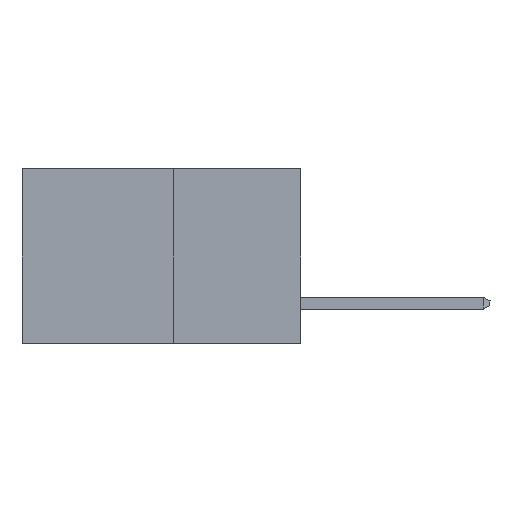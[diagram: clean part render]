
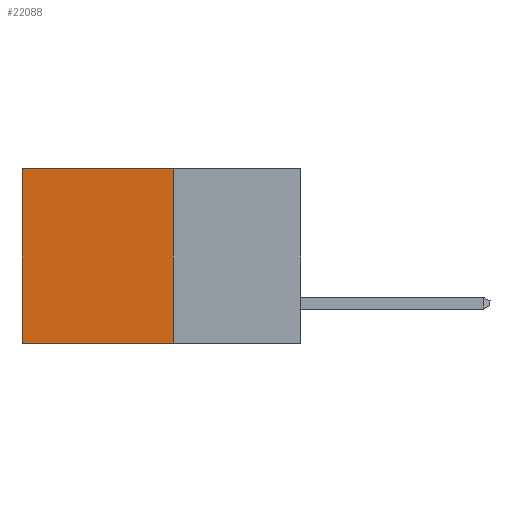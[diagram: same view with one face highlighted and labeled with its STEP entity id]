
A CAD part, left-side view. The second image highlights one B-rep face of the part: STEP entity #22088.
In plain terms, the highlighted planar face has unit normal (-1, 0, 0).
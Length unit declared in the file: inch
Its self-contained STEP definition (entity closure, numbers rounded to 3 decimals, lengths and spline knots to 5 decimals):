
#2346 = DIRECTION ( 'NONE',  ( 0., 0., -1. ) ) ;
#3459 = CARTESIAN_POINT ( 'NONE',  ( 0.277, 0.27, 0. ) ) ;
#5425 = CARTESIAN_POINT ( 'NONE',  ( 0.277, 0.59, -0.37 ) ) ;
#5531 = EDGE_CURVE ( 'NONE', #6152, #24925, #17665, .T. ) ;
#5925 = DIRECTION ( 'NONE',  ( 0., 1., 0. ) ) ;
#6152 = VERTEX_POINT ( 'NONE', #19104 ) ;
#6486 = DIRECTION ( 'NONE',  ( 0., 1., 0. ) ) ;
#6534 = CARTESIAN_POINT ( 'NONE',  ( 0.277, 0.27, -0.37 ) ) ;
#6620 = VERTEX_POINT ( 'NONE', #6926 ) ;
#6926 = CARTESIAN_POINT ( 'NONE',  ( 0.277, 0.59, 0. ) ) ;
#7099 = CARTESIAN_POINT ( 'NONE',  ( 0.277, 0.59, -0.37 ) ) ;
#8309 = CARTESIAN_POINT ( 'NONE',  ( 0.277, 0.27, -0.37 ) ) ;
#9009 = VECTOR ( 'NONE', #27202, 39.37008 ) ;
#9102 = EDGE_CURVE ( 'NONE', #6152, #6620, #20830, .T. ) ;
#10295 = EDGE_CURVE ( 'NONE', #6620, #13520, #28213, .T. ) ;
#10726 = DIRECTION ( 'NONE',  ( 0., 0., -1. ) ) ;
#12032 = EDGE_LOOP ( 'NONE', ( #17692, #26607, #27364, #13742 ) ) ;
#13520 = VERTEX_POINT ( 'NONE', #7099 ) ;
#13742 = ORIENTED_EDGE ( 'NONE', *, *, #9102, .T. ) ;
#15540 = PLANE ( 'NONE',  #15810 ) ;
#15810 = AXIS2_PLACEMENT_3D ( 'NONE', #8309, #25246, #10726 ) ;
#17665 = LINE ( 'NONE', #19442, #30303 ) ;
#17692 = ORIENTED_EDGE ( 'NONE', *, *, #10295, .T. ) ;
#19104 = CARTESIAN_POINT ( 'NONE',  ( 0.277, 0.27, 0. ) ) ;
#19442 = CARTESIAN_POINT ( 'NONE',  ( 0.277, 0.27, -0.37 ) ) ;
#20830 = LINE ( 'NONE', #3459, #25682 ) ;
#21081 = CARTESIAN_POINT ( 'NONE',  ( 0.277, 0.27, -0.37 ) ) ;
#22088 = ADVANCED_FACE ( 'NONE', ( #24748 ), #15540, .F. ) ;
#22337 = VECTOR ( 'NONE', #6486, 39.37008 ) ;
#24748 = FACE_OUTER_BOUND ( 'NONE', #12032, .T. ) ;
#24925 = VERTEX_POINT ( 'NONE', #6534 ) ;
#25246 = DIRECTION ( 'NONE',  ( 1., 0., 0. ) ) ;
#25682 = VECTOR ( 'NONE', #5925, 39.37008 ) ;
#26607 = ORIENTED_EDGE ( 'NONE', *, *, #28149, .F. ) ;
#27202 = DIRECTION ( 'NONE',  ( 0., 0., -1. ) ) ;
#27364 = ORIENTED_EDGE ( 'NONE', *, *, #5531, .F. ) ;
#27882 = LINE ( 'NONE', #21081, #22337 ) ;
#28149 = EDGE_CURVE ( 'NONE', #24925, #13520, #27882, .T. ) ;
#28213 = LINE ( 'NONE', #5425, #9009 ) ;
#30303 = VECTOR ( 'NONE', #2346, 39.37008 ) ;
